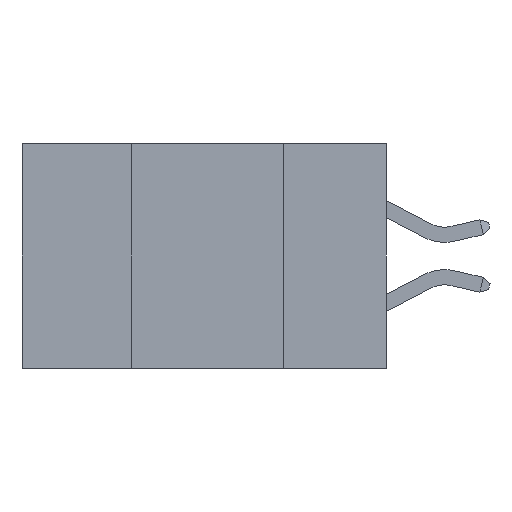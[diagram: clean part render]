
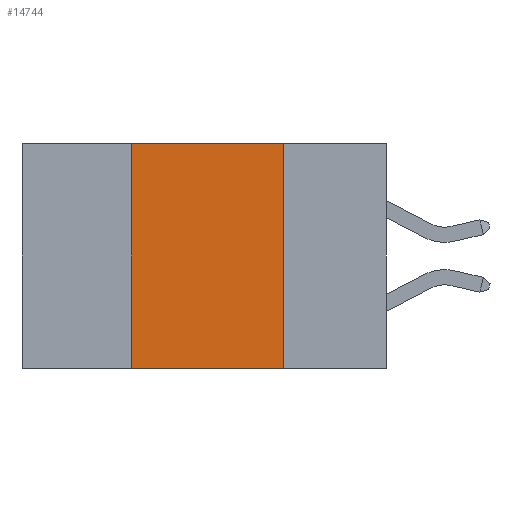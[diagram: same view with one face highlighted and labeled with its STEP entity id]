
A CAD part, left-side view. The second image highlights one B-rep face of the part: STEP entity #14744.
In plain terms, the highlighted planar face has unit normal (-1, 0, 0).
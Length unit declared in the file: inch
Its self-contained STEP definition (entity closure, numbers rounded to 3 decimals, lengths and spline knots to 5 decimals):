
#2141 = VERTEX_POINT ( 'NONE', #14703 ) ;
#2308 = EDGE_CURVE ( 'NONE', #2141, #18311, #14301, .T. ) ;
#2781 = VECTOR ( 'NONE', #7202, 39.37008 ) ;
#3739 = DIRECTION ( 'NONE',  ( 0., -1., 0. ) ) ;
#3869 = CARTESIAN_POINT ( 'NONE',  ( 0., 0.17, -0.37 ) ) ;
#3933 = CARTESIAN_POINT ( 'NONE',  ( 0., 0.6, 0. ) ) ;
#4395 = CARTESIAN_POINT ( 'NONE',  ( 0., 0.42, -0.37 ) ) ;
#6092 = ORIENTED_EDGE ( 'NONE', *, *, #15822, .F. ) ;
#6228 = EDGE_CURVE ( 'NONE', #2141, #17384, #15216, .T. ) ;
#6549 = VECTOR ( 'NONE', #20534, 39.37008 ) ;
#6917 = VECTOR ( 'NONE', #3739, 39.37008 ) ;
#7202 = DIRECTION ( 'NONE',  ( 0., 0., -1. ) ) ;
#7231 = LINE ( 'NONE', #3869, #2781 ) ;
#7879 = ORIENTED_EDGE ( 'NONE', *, *, #2308, .T. ) ;
#8930 = DIRECTION ( 'NONE',  ( 0., 0., -1. ) ) ;
#9527 = EDGE_CURVE ( 'NONE', #19242, #18311, #7231, .T. ) ;
#9853 = AXIS2_PLACEMENT_3D ( 'NONE', #3933, #18620, #8930 ) ;
#9969 = VECTOR ( 'NONE', #18922, 39.37008 ) ;
#10567 = CARTESIAN_POINT ( 'NONE',  ( 0., 0.42, 0. ) ) ;
#11834 = CARTESIAN_POINT ( 'NONE',  ( 0., 0.6, 0. ) ) ;
#12189 = ORIENTED_EDGE ( 'NONE', *, *, #6228, .F. ) ;
#12771 = CARTESIAN_POINT ( 'NONE',  ( 0., 0.17, -0.37 ) ) ;
#13129 = FACE_OUTER_BOUND ( 'NONE', #20171, .T. ) ;
#13969 = ORIENTED_EDGE ( 'NONE', *, *, #9527, .F. ) ;
#14301 = LINE ( 'NONE', #19080, #9969 ) ;
#14703 = CARTESIAN_POINT ( 'NONE',  ( 0., 0.42, -0.37 ) ) ;
#14744 = ADVANCED_FACE ( 'NONE', ( #13129 ), #17019, .F. ) ;
#15216 = LINE ( 'NONE', #4395, #6549 ) ;
#15573 = LINE ( 'NONE', #11834, #6917 ) ;
#15822 = EDGE_CURVE ( 'NONE', #17384, #19242, #15573, .T. ) ;
#17019 = PLANE ( 'NONE',  #9853 ) ;
#17384 = VERTEX_POINT ( 'NONE', #10567 ) ;
#18311 = VERTEX_POINT ( 'NONE', #12771 ) ;
#18620 = DIRECTION ( 'NONE',  ( 1., 0., 0. ) ) ;
#18922 = DIRECTION ( 'NONE',  ( 0., -1., 0. ) ) ;
#19080 = CARTESIAN_POINT ( 'NONE',  ( 0., 0.6, -0.37 ) ) ;
#19242 = VERTEX_POINT ( 'NONE', #20978 ) ;
#20171 = EDGE_LOOP ( 'NONE', ( #13969, #6092, #12189, #7879 ) ) ;
#20534 = DIRECTION ( 'NONE',  ( 0., 0., 1. ) ) ;
#20978 = CARTESIAN_POINT ( 'NONE',  ( 0., 0.17, 0. ) ) ;
